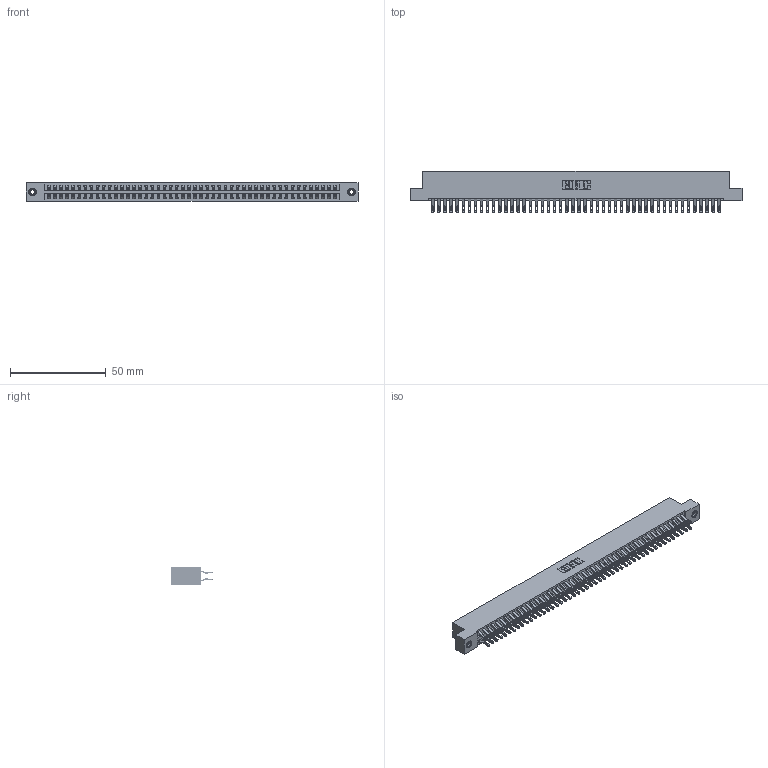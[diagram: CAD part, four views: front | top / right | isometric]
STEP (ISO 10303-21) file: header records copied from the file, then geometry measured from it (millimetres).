
FILE_DESCRIPTION (( 'STEP AP203' ), '1' );
FILE_NAME ('396-096-555-208.STEP', '2018-09-14T03:08:22', ( '' ), ( '' ), 'SwSTEP 2.0', 'SolidWorks 2016', '' );
FILE_SCHEMA (( 'CONFIG_CONTROL_DESIGN' ));
Length unit declared in the file: inch
Products named in the file (4): 345-292-001_555 Tail; 346 Part_Flush Mounting Lugs - 0.156 Dia-TI; 345-250-001_345-250-003-102; 396-096-555-208
Assembly tree (99 placements, depth 2):
  396-096-555-208
    346 Part_Flush Mounting Lugs - 0.156 Dia-TI
    345-292-001_555 Tail  x96
    345-250-001_345-250-003-102  x2
Bounding box: 172.97 x 21.46 x 9.4 mm (x, y, z)
Volume: 17185.6 mm3; surface area: 24729.7 mm2
Topology: 99 solids, 99 shells, 5750 faces, 18033 edges, 12014 vertices
Faces by surface type: plane 3276, cylinder 2458, cone 12, torus 4
Entity records: 32030 total; most frequent: CARTESIAN_POINT 5289, ORIENTED_EDGE 5186, DIRECTION 4707, EDGE_CURVE 2593, LINE 2229, VECTOR 2229, VERTEX_POINT 1724, AXIS2_PLACEMENT_3D 1239
